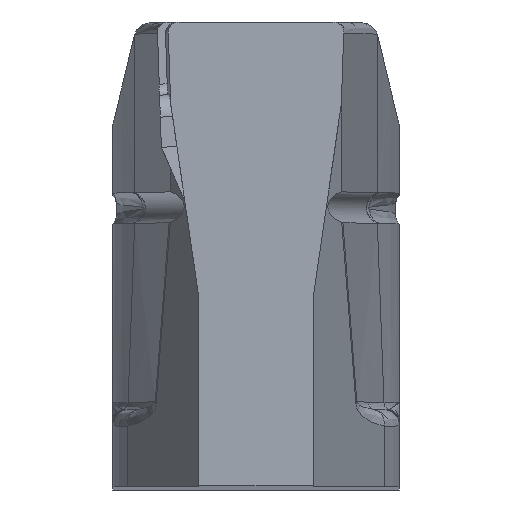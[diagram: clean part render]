
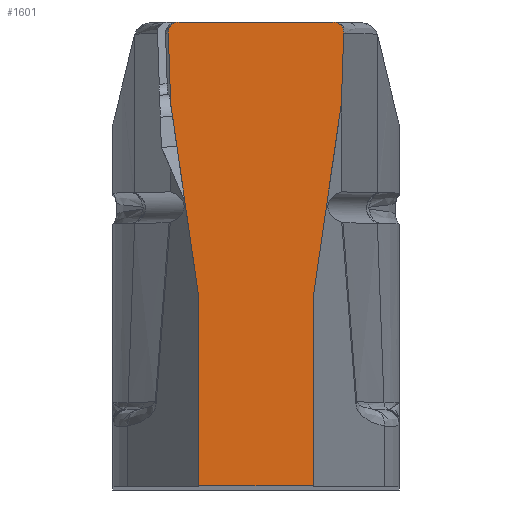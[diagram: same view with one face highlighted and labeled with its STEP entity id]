
A CAD part, top view. The second image highlights one B-rep face of the part: STEP entity #1601.
In plain terms, the highlighted planar face has unit normal (0, 0, 1).
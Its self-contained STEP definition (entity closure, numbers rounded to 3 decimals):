
#48=ELLIPSE('',#1727,0.691,0.689);
#49=ELLIPSE('',#1729,0.691,0.689);
#135=PLANE('',#1734);
#226=FACE_OUTER_BOUND('',#317,.T.);
#317=EDGE_LOOP('',(#1463,#1464,#1465,#1466,#1467,#1468,#1469,#1470,#1471,
#1472));
#345=LINE('',#2384,#452);
#350=LINE('',#2393,#457);
#413=LINE('',#4259,#520);
#415=LINE('',#4289,#522);
#418=LINE('',#4320,#525);
#420=LINE('',#4324,#527);
#422=LINE('',#4328,#529);
#424=LINE('',#4331,#531);
#452=VECTOR('',#1788,10.);
#457=VECTOR('',#1795,10.);
#520=VECTOR('',#2054,10.);
#522=VECTOR('',#2060,10.);
#525=VECTOR('',#2067,10.);
#527=VECTOR('',#2071,10.);
#529=VECTOR('',#2075,10.);
#531=VECTOR('',#2079,10.);
#625=VERTEX_POINT('',#2381);
#626=VERTEX_POINT('',#2383);
#629=VERTEX_POINT('',#2391);
#743=VERTEX_POINT('',#4257);
#744=VERTEX_POINT('',#4284);
#745=VERTEX_POINT('',#4288);
#746=VERTEX_POINT('',#4315);
#747=VERTEX_POINT('',#4319);
#748=VERTEX_POINT('',#4323);
#749=VERTEX_POINT('',#4327);
#789=EDGE_CURVE('',#626,#625,#345,.T.);
#794=EDGE_CURVE('',#625,#629,#350,.T.);
#977=EDGE_CURVE('',#629,#743,#413,.T.);
#978=EDGE_CURVE('',#744,#626,#48,.T.);
#980=EDGE_CURVE('',#745,#744,#415,.T.);
#982=EDGE_CURVE('',#746,#745,#49,.T.);
#984=EDGE_CURVE('',#747,#746,#418,.T.);
#986=EDGE_CURVE('',#748,#747,#420,.T.);
#988=EDGE_CURVE('',#749,#748,#422,.T.);
#990=EDGE_CURVE('',#743,#749,#424,.T.);
#1463=ORIENTED_EDGE('',*,*,#990,.T.);
#1464=ORIENTED_EDGE('',*,*,#988,.T.);
#1465=ORIENTED_EDGE('',*,*,#986,.T.);
#1466=ORIENTED_EDGE('',*,*,#984,.T.);
#1467=ORIENTED_EDGE('',*,*,#982,.T.);
#1468=ORIENTED_EDGE('',*,*,#980,.T.);
#1469=ORIENTED_EDGE('',*,*,#978,.T.);
#1470=ORIENTED_EDGE('',*,*,#789,.T.);
#1471=ORIENTED_EDGE('',*,*,#794,.T.);
#1472=ORIENTED_EDGE('',*,*,#977,.T.);
#1601=ADVANCED_FACE('',(#226),#135,.T.);
#1727=AXIS2_PLACEMENT_3D('',#4285,#2055,#2056);
#1729=AXIS2_PLACEMENT_3D('',#4316,#2062,#2063);
#1734=AXIS2_PLACEMENT_3D('',#4332,#2080,#2081);
#1788=DIRECTION('',(0.034,-0.999,0.));
#1795=DIRECTION('',(0.144,-0.99,0.));
#2054=DIRECTION('',(0.,-1.,0.));
#2055=DIRECTION('center_axis',(0.,0.,
1.));
#2056=DIRECTION('ref_axis',(1.,0.,0.));
#2060=DIRECTION('',(-1.,0.,0.));
#2062=DIRECTION('center_axis',(0.,0.,1.));
#2063=DIRECTION('ref_axis',(1.,0.,0.));
#2067=DIRECTION('',(0.034,0.999,0.));
#2071=DIRECTION('',(0.144,0.99,0.));
#2075=DIRECTION('',(0.,1.,0.));
#2079=DIRECTION('',(1.,0.,0.));
#2080=DIRECTION('center_axis',(0.,0.,1.));
#2081=DIRECTION('ref_axis',(1.,0.,0.));
#2381=CARTESIAN_POINT('',(-5.572,9.684,153.212));
#2383=CARTESIAN_POINT('',(-5.724,14.215,153.212));
#2384=CARTESIAN_POINT('',(-5.311,1.913,153.212));
#2391=CARTESIAN_POINT('',(-3.753,-2.837,153.212));
#2393=CARTESIAN_POINT('',(-3.628,-3.702,153.212));
#4257=CARTESIAN_POINT('',(-3.753,-14.872,153.212));
#4259=CARTESIAN_POINT('',(-3.753,-8.091,153.212));
#4284=CARTESIAN_POINT('',(-5.034,14.927,153.212));
#4285=CARTESIAN_POINT('Origin',(-5.034,14.238,153.212));
#4288=CARTESIAN_POINT('',(4.853,14.927,153.212));
#4289=CARTESIAN_POINT('',(7.829,14.927,153.212));
#4315=CARTESIAN_POINT('',(5.543,14.215,153.212));
#4316=CARTESIAN_POINT('Origin',(4.853,14.238,153.212));
#4319=CARTESIAN_POINT('',(5.391,9.684,153.212));
#4320=CARTESIAN_POINT('',(5.13,1.913,153.212));
#4323=CARTESIAN_POINT('',(3.573,-2.837,153.212));
#4324=CARTESIAN_POINT('',(3.447,-3.702,153.212));
#4327=CARTESIAN_POINT('',(3.573,-14.872,153.212));
#4328=CARTESIAN_POINT('',(3.573,-8.091,153.212));
#4331=CARTESIAN_POINT('',(0.107,-14.872,153.212));
#4332=CARTESIAN_POINT('Origin',(-0.091,-0.121,
153.212));
